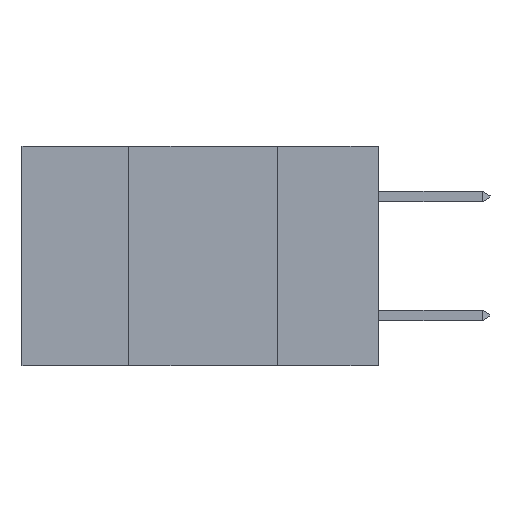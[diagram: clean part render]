
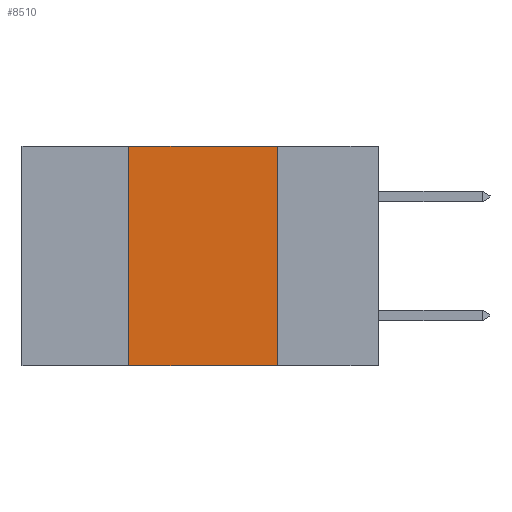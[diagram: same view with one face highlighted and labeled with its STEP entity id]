
A CAD part, left-side view. The second image highlights one B-rep face of the part: STEP entity #8510.
In plain terms, the highlighted planar face has unit normal (-1, 0, 0).
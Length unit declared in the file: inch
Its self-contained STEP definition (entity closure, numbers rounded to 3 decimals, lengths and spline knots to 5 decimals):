
#237 = LINE ( 'NONE', #7587, #1383 ) ;
#849 = DIRECTION ( 'NONE',  ( 0., 0., 1. ) ) ;
#853 = EDGE_CURVE ( 'NONE', #3570, #2871, #6797, .T. ) ;
#1189 = DIRECTION ( 'NONE',  ( 1., 0., 0. ) ) ;
#1202 = EDGE_CURVE ( 'NONE', #2871, #2920, #237, .T. ) ;
#1383 = VECTOR ( 'NONE', #9062, 39.37008 ) ;
#1692 = ORIENTED_EDGE ( 'NONE', *, *, #4933, .F. ) ;
#2091 = VECTOR ( 'NONE', #849, 39.37008 ) ;
#2647 = DIRECTION ( 'NONE',  ( 0., 0., -1. ) ) ;
#2871 = VERTEX_POINT ( 'NONE', #6996 ) ;
#2920 = VERTEX_POINT ( 'NONE', #6193 ) ;
#3029 = LINE ( 'NONE', #3128, #2091 ) ;
#3090 = DIRECTION ( 'NONE',  ( 0., -1., 0. ) ) ;
#3128 = CARTESIAN_POINT ( 'NONE',  ( 0., 0.42, -0.37 ) ) ;
#3162 = ORIENTED_EDGE ( 'NONE', *, *, #4276, .T. ) ;
#3570 = VERTEX_POINT ( 'NONE', #4434 ) ;
#4044 = VERTEX_POINT ( 'NONE', #8964 ) ;
#4063 = ORIENTED_EDGE ( 'NONE', *, *, #1202, .F. ) ;
#4276 = EDGE_CURVE ( 'NONE', #4044, #2920, #5810, .T. ) ;
#4434 = CARTESIAN_POINT ( 'NONE',  ( 0., 0.42, 0. ) ) ;
#4771 = CARTESIAN_POINT ( 'NONE',  ( 0., 0.6, 0. ) ) ;
#4887 = EDGE_LOOP ( 'NONE', ( #4063, #8007, #1692, #3162 ) ) ;
#4933 = EDGE_CURVE ( 'NONE', #4044, #3570, #3029, .T. ) ;
#4966 = VECTOR ( 'NONE', #7939, 39.37008 ) ;
#5378 = CARTESIAN_POINT ( 'NONE',  ( 0., 0.6, 0. ) ) ;
#5666 = CARTESIAN_POINT ( 'NONE',  ( 0., 0.6, -0.37 ) ) ;
#5810 = LINE ( 'NONE', #5666, #4966 ) ;
#6193 = CARTESIAN_POINT ( 'NONE',  ( 0., 0.17, -0.37 ) ) ;
#6539 = VECTOR ( 'NONE', #3090, 39.37008 ) ;
#6797 = LINE ( 'NONE', #5378, #6539 ) ;
#6878 = AXIS2_PLACEMENT_3D ( 'NONE', #4771, #1189, #2647 ) ;
#6996 = CARTESIAN_POINT ( 'NONE',  ( 0., 0.17, 0. ) ) ;
#7587 = CARTESIAN_POINT ( 'NONE',  ( 0., 0.17, -0.37 ) ) ;
#7939 = DIRECTION ( 'NONE',  ( 0., -1., 0. ) ) ;
#8007 = ORIENTED_EDGE ( 'NONE', *, *, #853, .F. ) ;
#8352 = FACE_OUTER_BOUND ( 'NONE', #4887, .T. ) ;
#8510 = ADVANCED_FACE ( 'NONE', ( #8352 ), #9083, .F. ) ;
#8964 = CARTESIAN_POINT ( 'NONE',  ( 0., 0.42, -0.37 ) ) ;
#9062 = DIRECTION ( 'NONE',  ( 0., 0., -1. ) ) ;
#9083 = PLANE ( 'NONE',  #6878 ) ;
